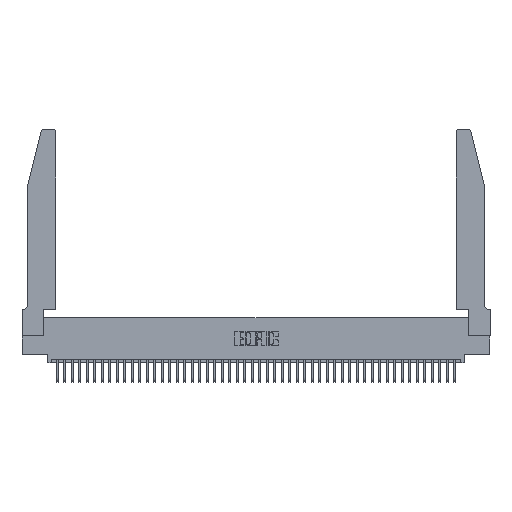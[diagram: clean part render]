
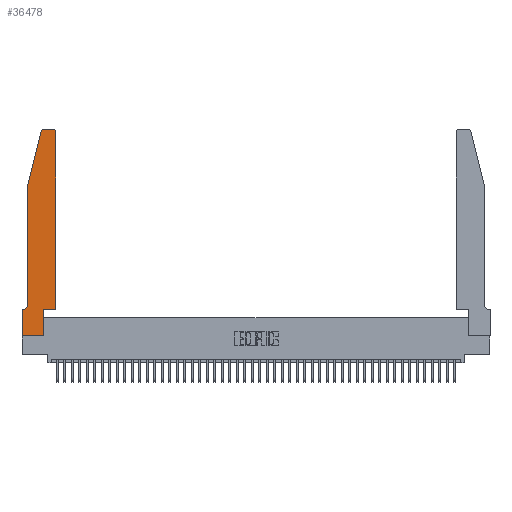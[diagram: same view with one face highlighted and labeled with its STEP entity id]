
A CAD part, top view. The second image highlights one B-rep face of the part: STEP entity #36478.
In plain terms, the highlighted planar face has unit normal (0, 0, 1).
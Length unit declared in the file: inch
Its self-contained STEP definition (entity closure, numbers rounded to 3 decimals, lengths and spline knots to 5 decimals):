
#2232 = EDGE_CURVE ( 'NONE', #34902, #16842, #27704, .T. ) ;
#2636 = CARTESIAN_POINT ( 'NONE',  ( 0.4505, 0.35, 0.37 ) ) ;
#2779 = VERTEX_POINT ( 'NONE', #29628 ) ;
#2784 = AXIS2_PLACEMENT_3D ( 'NONE', #39946, #19630, #43346 ) ;
#3332 = CARTESIAN_POINT ( 'NONE',  ( 0., 0.35, 0.37 ) ) ;
#3531 = EDGE_CURVE ( 'NONE', #29058, #34902, #32896, .T. ) ;
#3702 = CARTESIAN_POINT ( 'NONE',  ( 0.25487, 2.72718, 0.37 ) ) ;
#4848 = LINE ( 'NONE', #14508, #21842 ) ;
#6055 = VECTOR ( 'NONE', #18289, 39.37008 ) ;
#6693 = VERTEX_POINT ( 'NONE', #31026 ) ;
#6768 = DIRECTION ( 'NONE',  ( 0., 0., 1. ) ) ;
#7640 = VECTOR ( 'NONE', #26838, 39.37008 ) ;
#7820 = LINE ( 'NONE', #2636, #15755 ) ;
#8007 = LINE ( 'NONE', #13465, #41943 ) ;
#8117 = EDGE_CURVE ( 'NONE', #29275, #20023, #21702, .T. ) ;
#8394 = FACE_OUTER_BOUND ( 'NONE', #27182, .T. ) ;
#8411 = DIRECTION ( 'NONE',  ( 0., 0., -1. ) ) ;
#8722 = DIRECTION ( 'NONE',  ( 0., -1., 0. ) ) ;
#8988 = VERTEX_POINT ( 'NONE', #35480 ) ;
#9146 = AXIS2_PLACEMENT_3D ( 'NONE', #13025, #36757, #16454 ) ;
#10326 = EDGE_CURVE ( 'NONE', #20023, #20833, #18772, .T. ) ;
#12173 = AXIS2_PLACEMENT_3D ( 'NONE', #28733, #8411, #32128 ) ;
#12259 = DIRECTION ( 'NONE',  ( 0., -1., 0. ) ) ;
#12616 = VECTOR ( 'NONE', #12259, 39.37008 ) ;
#13025 = CARTESIAN_POINT ( 'NONE',  ( 0.284, 2.72, 0.37 ) ) ;
#13029 = EDGE_CURVE ( 'NONE', #6693, #24681, #34697, .T. ) ;
#13216 = CARTESIAN_POINT ( 'NONE',  ( 0.2605, 2.75, 0.37 ) ) ;
#13465 = CARTESIAN_POINT ( 'NONE',  ( 0.0755, 2., 0.37 ) ) ;
#13972 = LINE ( 'NONE', #42018, #6055 ) ;
#14508 = CARTESIAN_POINT ( 'NONE',  ( 0., 0., 0.37 ) ) ;
#15755 = VECTOR ( 'NONE', #23762, 39.37008 ) ;
#15925 = VECTOR ( 'NONE', #23454, 39.37008 ) ;
#16426 = AXIS2_PLACEMENT_3D ( 'NONE', #3332, #6768, #30494 ) ;
#16454 = DIRECTION ( 'NONE',  ( 1., 0., 0. ) ) ;
#16745 = CARTESIAN_POINT ( 'NONE',  ( 0.0755, 0.35, 0.37 ) ) ;
#16761 = EDGE_CURVE ( 'NONE', #2779, #30070, #7820, .T. ) ;
#16842 = VERTEX_POINT ( 'NONE', #3702 ) ;
#17923 = DIRECTION ( 'NONE',  ( 1., 0., 0. ) ) ;
#18052 = LINE ( 'NONE', #16745, #15925 ) ;
#18196 = CARTESIAN_POINT ( 'NONE',  ( 0.4205, 2.75, 0.37 ) ) ;
#18289 = DIRECTION ( 'NONE',  ( 1., 0., 0. ) ) ;
#18772 = CIRCLE ( 'NONE', #12173, 0.07 ) ;
#18870 = ORIENTED_EDGE ( 'NONE', *, *, #3531, .T. ) ;
#18962 = CARTESIAN_POINT ( 'NONE',  ( 0.0755, 2., 0.37 ) ) ;
#19494 = ORIENTED_EDGE ( 'NONE', *, *, #29181, .T. ) ;
#19630 = DIRECTION ( 'NONE',  ( 0., 0., 1. ) ) ;
#20023 = VERTEX_POINT ( 'NONE', #34557 ) ;
#20074 = EDGE_CURVE ( 'NONE', #39984, #6693, #4848, .T. ) ;
#20833 = VERTEX_POINT ( 'NONE', #22076 ) ;
#21702 = LINE ( 'NONE', #18962, #12616 ) ;
#21842 = VECTOR ( 'NONE', #17923, 39.37008 ) ;
#22076 = CARTESIAN_POINT ( 'NONE',  ( 0.0055, 0.35, 0.37 ) ) ;
#23428 = CARTESIAN_POINT ( 'NONE',  ( 0.2865, 0.35, 0.37 ) ) ;
#23454 = DIRECTION ( 'NONE',  ( -1., 0., 0. ) ) ;
#23692 = PLANE ( 'NONE',  #16426 ) ;
#23762 = DIRECTION ( 'NONE',  ( 0., 1., 0. ) ) ;
#23784 = CARTESIAN_POINT ( 'NONE',  ( 0.4505, 2.72, 0.37 ) ) ;
#23882 = VECTOR ( 'NONE', #40376, 39.37008 ) ;
#24635 = EDGE_CURVE ( 'NONE', #30070, #29058, #26614, .T. ) ;
#24681 = VERTEX_POINT ( 'NONE', #36666 ) ;
#26442 = CARTESIAN_POINT ( 'NONE',  ( 0., 0., 0.37 ) ) ;
#26614 = CIRCLE ( 'NONE', #2784, 0.03 ) ;
#26714 = LINE ( 'NONE', #32295, #42602 ) ;
#26838 = DIRECTION ( 'NONE',  ( 0., 1., 0. ) ) ;
#27182 = EDGE_LOOP ( 'NONE', ( #18870, #40882, #43119, #40480, #38058, #42435, #19494, #41996, #39083, #30583, #30343, #32843 ) ) ;
#27704 = CIRCLE ( 'NONE', #9146, 0.03 ) ;
#28733 = CARTESIAN_POINT ( 'NONE',  ( 0.0055, 0.42, 0.37 ) ) ;
#29058 = VERTEX_POINT ( 'NONE', #18196 ) ;
#29181 = EDGE_CURVE ( 'NONE', #8988, #39984, #26714, .T. ) ;
#29275 = VERTEX_POINT ( 'NONE', #32884 ) ;
#29628 = CARTESIAN_POINT ( 'NONE',  ( 0.4505, 0.35, 0.37 ) ) ;
#30070 = VERTEX_POINT ( 'NONE', #23784 ) ;
#30343 = ORIENTED_EDGE ( 'NONE', *, *, #16761, .T. ) ;
#30397 = DIRECTION ( 'NONE',  ( -0.239, -0.971, 0. ) ) ;
#30494 = DIRECTION ( 'NONE',  ( 1., 0., 0. ) ) ;
#30583 = ORIENTED_EDGE ( 'NONE', *, *, #35042, .T. ) ;
#30612 = EDGE_CURVE ( 'NONE', #20833, #8988, #18052, .T. ) ;
#31026 = CARTESIAN_POINT ( 'NONE',  ( 0.2865, 0., 0.37 ) ) ;
#31324 = EDGE_CURVE ( 'NONE', #16842, #29275, #8007, .T. ) ;
#32128 = DIRECTION ( 'NONE',  ( -1., 0., 0. ) ) ;
#32295 = CARTESIAN_POINT ( 'NONE',  ( 0., 0., 0.37 ) ) ;
#32843 = ORIENTED_EDGE ( 'NONE', *, *, #24635, .T. ) ;
#32884 = CARTESIAN_POINT ( 'NONE',  ( 0.0755, 2., 0.37 ) ) ;
#32896 = LINE ( 'NONE', #13216, #23882 ) ;
#34469 = CARTESIAN_POINT ( 'NONE',  ( 0.284, 2.75, 0.37 ) ) ;
#34557 = CARTESIAN_POINT ( 'NONE',  ( 0.0755, 0.42, 0.37 ) ) ;
#34697 = LINE ( 'NONE', #23428, #7640 ) ;
#34902 = VERTEX_POINT ( 'NONE', #34469 ) ;
#35042 = EDGE_CURVE ( 'NONE', #24681, #2779, #13972, .T. ) ;
#35480 = CARTESIAN_POINT ( 'NONE',  ( 0., 0.35, 0.37 ) ) ;
#36478 = ADVANCED_FACE ( 'NONE', ( #8394 ), #23692, .T. ) ;
#36666 = CARTESIAN_POINT ( 'NONE',  ( 0.2865, 0.35, 0.37 ) ) ;
#36757 = DIRECTION ( 'NONE',  ( 0., 0., 1. ) ) ;
#38058 = ORIENTED_EDGE ( 'NONE', *, *, #10326, .T. ) ;
#39083 = ORIENTED_EDGE ( 'NONE', *, *, #13029, .T. ) ;
#39946 = CARTESIAN_POINT ( 'NONE',  ( 0.4205, 2.72, 0.37 ) ) ;
#39984 = VERTEX_POINT ( 'NONE', #26442 ) ;
#40376 = DIRECTION ( 'NONE',  ( -1., 0., 0. ) ) ;
#40480 = ORIENTED_EDGE ( 'NONE', *, *, #8117, .T. ) ;
#40882 = ORIENTED_EDGE ( 'NONE', *, *, #2232, .T. ) ;
#41943 = VECTOR ( 'NONE', #30397, 39.37008 ) ;
#41996 = ORIENTED_EDGE ( 'NONE', *, *, #20074, .T. ) ;
#42018 = CARTESIAN_POINT ( 'NONE',  ( 0.4505, 0.35, 0.37 ) ) ;
#42435 = ORIENTED_EDGE ( 'NONE', *, *, #30612, .T. ) ;
#42602 = VECTOR ( 'NONE', #8722, 39.37008 ) ;
#43119 = ORIENTED_EDGE ( 'NONE', *, *, #31324, .T. ) ;
#43346 = DIRECTION ( 'NONE',  ( 1., 0., 0. ) ) ;
